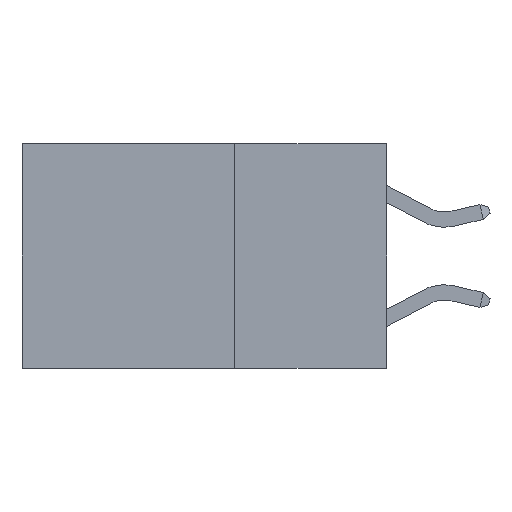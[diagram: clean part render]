
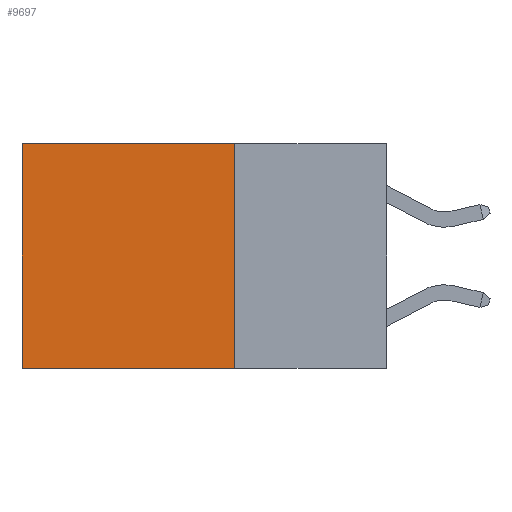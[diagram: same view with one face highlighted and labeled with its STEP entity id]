
A CAD part, left-side view. The second image highlights one B-rep face of the part: STEP entity #9697.
In plain terms, the highlighted planar face has unit normal (-1, 0, 0).
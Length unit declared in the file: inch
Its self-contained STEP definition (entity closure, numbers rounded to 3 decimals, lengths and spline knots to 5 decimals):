
#358 = CARTESIAN_POINT ( 'NONE',  ( 0.2625, 0.25, 0. ) ) ;
#1095 = FACE_OUTER_BOUND ( 'NONE', #5962, .T. ) ;
#1119 = EDGE_CURVE ( 'NONE', #5265, #8697, #1495, .T. ) ;
#1421 = DIRECTION ( 'NONE',  ( 0., 1., 0. ) ) ;
#1495 = LINE ( 'NONE', #5913, #3821 ) ;
#1840 = EDGE_CURVE ( 'NONE', #8697, #3865, #4078, .T. ) ;
#2154 = DIRECTION ( 'NONE',  ( 1., 0., 0. ) ) ;
#2834 = CARTESIAN_POINT ( 'NONE',  ( 0.2625, 0.6, -0.37 ) ) ;
#3489 = PLANE ( 'NONE',  #5981 ) ;
#3821 = VECTOR ( 'NONE', #1421, 39.37008 ) ;
#3865 = VERTEX_POINT ( 'NONE', #2834 ) ;
#4078 = LINE ( 'NONE', #9751, #9347 ) ;
#4153 = CARTESIAN_POINT ( 'NONE',  ( 0.2625, 0.25, 0. ) ) ;
#4354 = LINE ( 'NONE', #12021, #13525 ) ;
#5265 = VERTEX_POINT ( 'NONE', #4153 ) ;
#5581 = DIRECTION ( 'NONE',  ( 0., 0., -1. ) ) ;
#5913 = CARTESIAN_POINT ( 'NONE',  ( 0.2625, 0.25, 0. ) ) ;
#5962 = EDGE_LOOP ( 'NONE', ( #11206, #10746, #6451, #8136 ) ) ;
#5981 = AXIS2_PLACEMENT_3D ( 'NONE', #13098, #2154, #5581 ) ;
#6451 = ORIENTED_EDGE ( 'NONE', *, *, #10521, .F. ) ;
#6603 = DIRECTION ( 'NONE',  ( 0., 0., -1. ) ) ;
#7078 = CARTESIAN_POINT ( 'NONE',  ( 0.2625, 0.6, 0. ) ) ;
#8136 = ORIENTED_EDGE ( 'NONE', *, *, #1119, .T. ) ;
#8593 = EDGE_CURVE ( 'NONE', #10068, #3865, #4354, .T. ) ;
#8697 = VERTEX_POINT ( 'NONE', #7078 ) ;
#8896 = DIRECTION ( 'NONE',  ( 0., 1., 0. ) ) ;
#9126 = VECTOR ( 'NONE', #6603, 39.37008 ) ;
#9347 = VECTOR ( 'NONE', #10824, 39.37008 ) ;
#9697 = ADVANCED_FACE ( 'NONE', ( #1095 ), #3489, .F. ) ;
#9751 = CARTESIAN_POINT ( 'NONE',  ( 0.2625, 0.6, 0. ) ) ;
#10068 = VERTEX_POINT ( 'NONE', #13724 ) ;
#10521 = EDGE_CURVE ( 'NONE', #5265, #10068, #10970, .T. ) ;
#10746 = ORIENTED_EDGE ( 'NONE', *, *, #8593, .F. ) ;
#10824 = DIRECTION ( 'NONE',  ( 0., 0., -1. ) ) ;
#10970 = LINE ( 'NONE', #358, #9126 ) ;
#11206 = ORIENTED_EDGE ( 'NONE', *, *, #1840, .T. ) ;
#12021 = CARTESIAN_POINT ( 'NONE',  ( 0.2625, 0.25, -0.37 ) ) ;
#13098 = CARTESIAN_POINT ( 'NONE',  ( 0.2625, 0.25, 0. ) ) ;
#13525 = VECTOR ( 'NONE', #8896, 39.37008 ) ;
#13724 = CARTESIAN_POINT ( 'NONE',  ( 0.2625, 0.25, -0.37 ) ) ;
